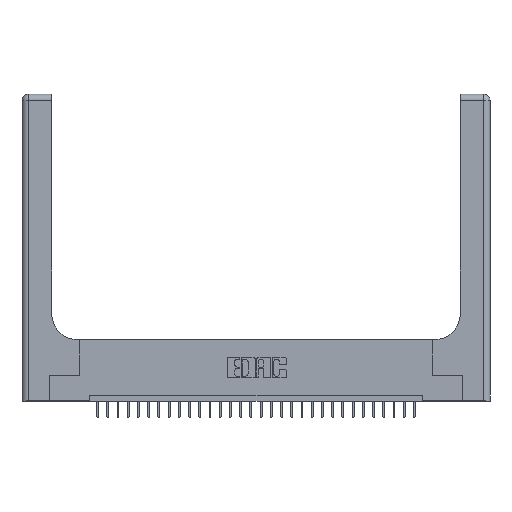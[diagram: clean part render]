
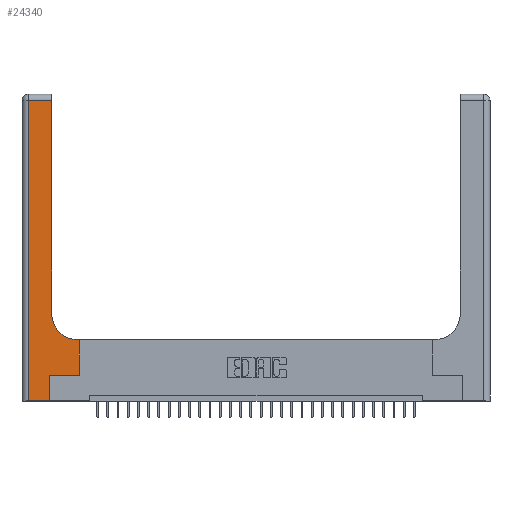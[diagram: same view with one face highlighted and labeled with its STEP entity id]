
A CAD part, top view. The second image highlights one B-rep face of the part: STEP entity #24340.
In plain terms, the highlighted planar face has unit normal (0, 0, 1).
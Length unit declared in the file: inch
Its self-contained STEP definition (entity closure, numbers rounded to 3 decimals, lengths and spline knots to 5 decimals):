
#97 = CARTESIAN_POINT ( 'NONE',  ( 0., 2.94, 0.37 ) ) ;
#265 = DIRECTION ( 'NONE',  ( -1., 0., 0. ) ) ;
#462 = DIRECTION ( 'NONE',  ( 0., -1., 0. ) ) ;
#478 = VECTOR ( 'NONE', #17350, 39.37008 ) ;
#959 = DIRECTION ( 'NONE',  ( 1., 0., 0. ) ) ;
#1698 = CARTESIAN_POINT ( 'NONE',  ( 0.5585, 0.6, 0.37 ) ) ;
#2209 = ORIENTED_EDGE ( 'NONE', *, *, #15151, .T. ) ;
#2264 = CARTESIAN_POINT ( 'NONE',  ( 0.269, 0., 0.37 ) ) ;
#2329 = CARTESIAN_POINT ( 'NONE',  ( 0.269, 0.25, 0.37 ) ) ;
#2832 = CARTESIAN_POINT ( 'NONE',  ( 0., 0., 0.37 ) ) ;
#2892 = DIRECTION ( 'NONE',  ( 0., 1., 0. ) ) ;
#3363 = VECTOR ( 'NONE', #12035, 39.37008 ) ;
#3671 = CARTESIAN_POINT ( 'NONE',  ( 0.5585, 0.25, 0.37 ) ) ;
#3750 = LINE ( 'NONE', #97, #478 ) ;
#4754 = CARTESIAN_POINT ( 'NONE',  ( 0.06, 3., 0.37 ) ) ;
#4788 = CARTESIAN_POINT ( 'NONE',  ( 0.269, 0.25, 0.37 ) ) ;
#5648 = EDGE_CURVE ( 'NONE', #11258, #23679, #10179, .T. ) ;
#6134 = VECTOR ( 'NONE', #2892, 39.37008 ) ;
#8140 = EDGE_CURVE ( 'NONE', #30583, #23280, #8526, .T. ) ;
#8526 = LINE ( 'NONE', #2329, #28205 ) ;
#8620 = CARTESIAN_POINT ( 'NONE',  ( 0.5585, 0.25, 0.37 ) ) ;
#8841 = CARTESIAN_POINT ( 'NONE',  ( 0.2915, 0.6, 0.37 ) ) ;
#9641 = CARTESIAN_POINT ( 'NONE',  ( 0., 3., 0.37 ) ) ;
#9658 = DIRECTION ( 'NONE',  ( 0., 1., 0. ) ) ;
#9715 = ORIENTED_EDGE ( 'NONE', *, *, #29475, .T. ) ;
#10055 = EDGE_CURVE ( 'NONE', #23280, #27994, #18455, .T. ) ;
#10179 = LINE ( 'NONE', #17481, #6134 ) ;
#10233 = EDGE_CURVE ( 'NONE', #14163, #17237, #22565, .T. ) ;
#11208 = CARTESIAN_POINT ( 'NONE',  ( 0.06, 0., 0.37 ) ) ;
#11258 = VERTEX_POINT ( 'NONE', #27809 ) ;
#12035 = DIRECTION ( 'NONE',  ( 1., 0., 0. ) ) ;
#12388 = VERTEX_POINT ( 'NONE', #16397 ) ;
#12497 = VECTOR ( 'NONE', #462, 39.37008 ) ;
#13045 = VECTOR ( 'NONE', #9658, 39.37008 ) ;
#13204 = ORIENTED_EDGE ( 'NONE', *, *, #10233, .T. ) ;
#13242 = LINE ( 'NONE', #8841, #16209 ) ;
#13307 = CARTESIAN_POINT ( 'NONE',  ( 0.2915, 2.94, 0.37 ) ) ;
#13576 = ORIENTED_EDGE ( 'NONE', *, *, #5648, .T. ) ;
#14163 = VERTEX_POINT ( 'NONE', #29806 ) ;
#15151 = EDGE_CURVE ( 'NONE', #23679, #14163, #3750, .T. ) ;
#15677 = EDGE_CURVE ( 'NONE', #17237, #28735, #19674, .T. ) ;
#16209 = VECTOR ( 'NONE', #30213, 39.37008 ) ;
#16397 = CARTESIAN_POINT ( 'NONE',  ( 0.5415, 0.6, 0.37 ) ) ;
#17237 = VERTEX_POINT ( 'NONE', #11208 ) ;
#17350 = DIRECTION ( 'NONE',  ( -1., 0., 0. ) ) ;
#17481 = CARTESIAN_POINT ( 'NONE',  ( 0.2915, 3., 0.37 ) ) ;
#18455 = LINE ( 'NONE', #8620, #20700 ) ;
#18877 = DIRECTION ( 'NONE',  ( 1., 0., 0. ) ) ;
#19184 = DIRECTION ( 'NONE',  ( 0., 0., -1. ) ) ;
#19294 = ORIENTED_EDGE ( 'NONE', *, *, #20395, .T. ) ;
#19674 = LINE ( 'NONE', #2832, #3363 ) ;
#20061 = ORIENTED_EDGE ( 'NONE', *, *, #15677, .T. ) ;
#20064 = CIRCLE ( 'NONE', #24938, 0.25 ) ;
#20395 = EDGE_CURVE ( 'NONE', #27994, #12388, #13242, .T. ) ;
#20441 = DIRECTION ( 'NONE',  ( 0., 1., 0. ) ) ;
#20700 = VECTOR ( 'NONE', #20441, 39.37008 ) ;
#21896 = CARTESIAN_POINT ( 'NONE',  ( 0.269, 0., 0.37 ) ) ;
#22132 = AXIS2_PLACEMENT_3D ( 'NONE', #9641, #19184, #265 ) ;
#22565 = LINE ( 'NONE', #4754, #12497 ) ;
#22905 = EDGE_LOOP ( 'NONE', ( #13576, #2209, #13204, #20061, #30347, #24746, #23855, #19294, #9715 ) ) ;
#23280 = VERTEX_POINT ( 'NONE', #3671 ) ;
#23462 = EDGE_CURVE ( 'NONE', #28735, #30583, #27190, .T. ) ;
#23679 = VERTEX_POINT ( 'NONE', #13307 ) ;
#23855 = ORIENTED_EDGE ( 'NONE', *, *, #10055, .T. ) ;
#24340 = ADVANCED_FACE ( 'NONE', ( #24556 ), #26170, .F. ) ;
#24556 = FACE_OUTER_BOUND ( 'NONE', #22905, .T. ) ;
#24746 = ORIENTED_EDGE ( 'NONE', *, *, #8140, .T. ) ;
#24938 = AXIS2_PLACEMENT_3D ( 'NONE', #29631, #26952, #959 ) ;
#26170 = PLANE ( 'NONE',  #22132 ) ;
#26952 = DIRECTION ( 'NONE',  ( 0., 0., -1. ) ) ;
#27190 = LINE ( 'NONE', #21896, #13045 ) ;
#27809 = CARTESIAN_POINT ( 'NONE',  ( 0.2915, 0.85, 0.37 ) ) ;
#27994 = VERTEX_POINT ( 'NONE', #1698 ) ;
#28205 = VECTOR ( 'NONE', #18877, 39.37008 ) ;
#28735 = VERTEX_POINT ( 'NONE', #2264 ) ;
#29475 = EDGE_CURVE ( 'NONE', #12388, #11258, #20064, .T. ) ;
#29631 = CARTESIAN_POINT ( 'NONE',  ( 0.5415, 0.85, 0.37 ) ) ;
#29806 = CARTESIAN_POINT ( 'NONE',  ( 0.06, 2.94, 0.37 ) ) ;
#30213 = DIRECTION ( 'NONE',  ( -1., 0., 0. ) ) ;
#30347 = ORIENTED_EDGE ( 'NONE', *, *, #23462, .T. ) ;
#30583 = VERTEX_POINT ( 'NONE', #4788 ) ;
